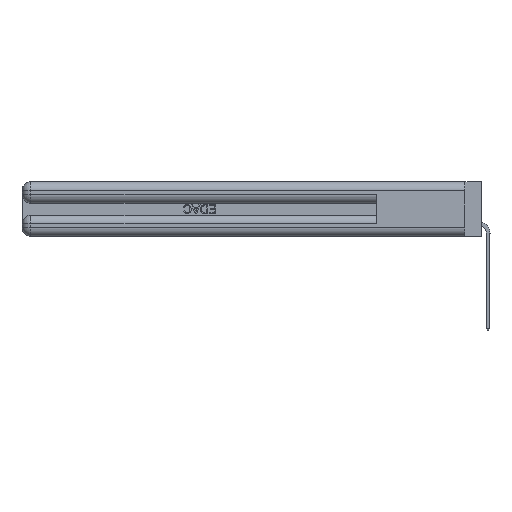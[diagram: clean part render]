
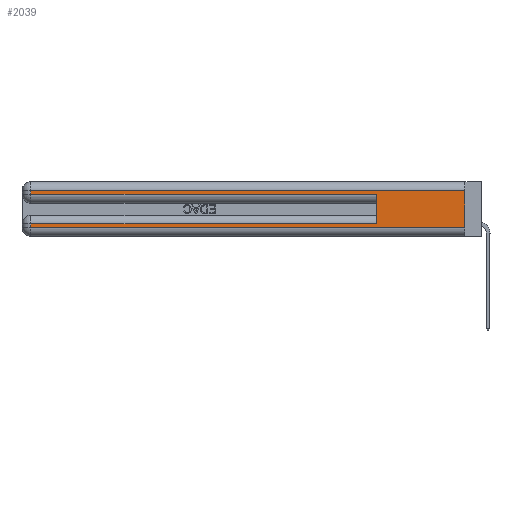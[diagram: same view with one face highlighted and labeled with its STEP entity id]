
A CAD part, left-side view. The second image highlights one B-rep face of the part: STEP entity #2039.
In plain terms, the highlighted planar face has unit normal (-1, 0, 0).
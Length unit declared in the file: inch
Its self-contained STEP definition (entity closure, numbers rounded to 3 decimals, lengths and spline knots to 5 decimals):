
#1283 = LINE ( 'NONE', #32755, #19797 ) ;
#1844 = EDGE_CURVE ( 'NONE', #20080, #29678, #5288, .T. ) ;
#2012 = DIRECTION ( 'NONE',  ( 0., 0., -1. ) ) ;
#2039 = ADVANCED_FACE ( 'NONE', ( #39711 ), #11212, .F. ) ;
#4358 = DIRECTION ( 'NONE',  ( 0., 1., 0. ) ) ;
#4381 = CARTESIAN_POINT ( 'NONE',  ( 0., 0., 0.285 ) ) ;
#4842 = LINE ( 'NONE', #4381, #40306 ) ;
#5288 = LINE ( 'NONE', #8274, #23747 ) ;
#5434 = EDGE_LOOP ( 'NONE', ( #35543, #8262, #37528, #19134, #39429, #38840, #17366, #28335 ) ) ;
#5841 = EDGE_CURVE ( 'NONE', #9917, #28536, #8396, .T. ) ;
#5960 = EDGE_CURVE ( 'NONE', #37163, #29678, #21373, .T. ) ;
#6861 = DIRECTION ( 'NONE',  ( 0., 0., -1. ) ) ;
#7276 = CARTESIAN_POINT ( 'NONE',  ( 0., 2.94, 0.37 ) ) ;
#8252 = CARTESIAN_POINT ( 'NONE',  ( 0., 2.94, 0.37 ) ) ;
#8262 = ORIENTED_EDGE ( 'NONE', *, *, #12371, .T. ) ;
#8274 = CARTESIAN_POINT ( 'NONE',  ( 0., 0., 0.37 ) ) ;
#8396 = LINE ( 'NONE', #16220, #25393 ) ;
#8474 = CARTESIAN_POINT ( 'NONE',  ( 0., 2.94, 0.06 ) ) ;
#9917 = VERTEX_POINT ( 'NONE', #32937 ) ;
#10785 = CARTESIAN_POINT ( 'NONE',  ( 0., 0., 0.31 ) ) ;
#11212 = PLANE ( 'NONE',  #32061 ) ;
#11316 = EDGE_CURVE ( 'NONE', #12801, #26693, #35589, .T. ) ;
#12371 = EDGE_CURVE ( 'NONE', #20080, #12801, #40641, .T. ) ;
#12664 = DIRECTION ( 'NONE',  ( 0., 0., -1. ) ) ;
#12801 = VERTEX_POINT ( 'NONE', #35189 ) ;
#15765 = CARTESIAN_POINT ( 'NONE',  ( 0., 0., 0.31 ) ) ;
#15889 = EDGE_CURVE ( 'NONE', #26693, #28536, #4842, .T. ) ;
#16038 = EDGE_CURVE ( 'NONE', #9917, #33114, #1283, .T. ) ;
#16220 = CARTESIAN_POINT ( 'NONE',  ( 0., 0.6, 0.145 ) ) ;
#17366 = ORIENTED_EDGE ( 'NONE', *, *, #32618, .T. ) ;
#18752 = VECTOR ( 'NONE', #6861, 39.37008 ) ;
#19134 = ORIENTED_EDGE ( 'NONE', *, *, #15889, .T. ) ;
#19797 = VECTOR ( 'NONE', #39759, 39.37008 ) ;
#20080 = VERTEX_POINT ( 'NONE', #15765 ) ;
#21373 = LINE ( 'NONE', #23965, #34326 ) ;
#22439 = CARTESIAN_POINT ( 'NONE',  ( 0., 0., 0.37 ) ) ;
#23747 = VECTOR ( 'NONE', #2012, 39.37008 ) ;
#23965 = CARTESIAN_POINT ( 'NONE',  ( 0., 0., 0.06 ) ) ;
#24268 = LINE ( 'NONE', #8252, #25289 ) ;
#24908 = DIRECTION ( 'NONE',  ( 1., 0., 0. ) ) ;
#25289 = VECTOR ( 'NONE', #36691, 39.37008 ) ;
#25393 = VECTOR ( 'NONE', #31012, 39.37008 ) ;
#26093 = CARTESIAN_POINT ( 'NONE',  ( 0., 0., 0.06 ) ) ;
#26693 = VERTEX_POINT ( 'NONE', #39604 ) ;
#28335 = ORIENTED_EDGE ( 'NONE', *, *, #5960, .T. ) ;
#28536 = VERTEX_POINT ( 'NONE', #28780 ) ;
#28780 = CARTESIAN_POINT ( 'NONE',  ( 0., 0.6, 0.285 ) ) ;
#29539 = CARTESIAN_POINT ( 'NONE',  ( 0., 2.94, 0.085 ) ) ;
#29678 = VERTEX_POINT ( 'NONE', #26093 ) ;
#30105 = DIRECTION ( 'NONE',  ( 0., -1., 0. ) ) ;
#30904 = DIRECTION ( 'NONE',  ( 0., -1., 0. ) ) ;
#31012 = DIRECTION ( 'NONE',  ( 0., 0., 1. ) ) ;
#32061 = AXIS2_PLACEMENT_3D ( 'NONE', #22439, #24908, #12664 ) ;
#32096 = VECTOR ( 'NONE', #4358, 39.37008 ) ;
#32618 = EDGE_CURVE ( 'NONE', #33114, #37163, #24268, .T. ) ;
#32755 = CARTESIAN_POINT ( 'NONE',  ( 0., 0., 0.085 ) ) ;
#32937 = CARTESIAN_POINT ( 'NONE',  ( 0., 0.6, 0.085 ) ) ;
#33114 = VERTEX_POINT ( 'NONE', #29539 ) ;
#34326 = VECTOR ( 'NONE', #30105, 39.37008 ) ;
#35189 = CARTESIAN_POINT ( 'NONE',  ( 0., 2.94, 0.31 ) ) ;
#35543 = ORIENTED_EDGE ( 'NONE', *, *, #1844, .F. ) ;
#35589 = LINE ( 'NONE', #7276, #18752 ) ;
#36691 = DIRECTION ( 'NONE',  ( 0., 0., -1. ) ) ;
#37163 = VERTEX_POINT ( 'NONE', #8474 ) ;
#37528 = ORIENTED_EDGE ( 'NONE', *, *, #11316, .T. ) ;
#38840 = ORIENTED_EDGE ( 'NONE', *, *, #16038, .T. ) ;
#39429 = ORIENTED_EDGE ( 'NONE', *, *, #5841, .F. ) ;
#39604 = CARTESIAN_POINT ( 'NONE',  ( 0., 2.94, 0.285 ) ) ;
#39711 = FACE_OUTER_BOUND ( 'NONE', #5434, .T. ) ;
#39759 = DIRECTION ( 'NONE',  ( 0., 1., 0. ) ) ;
#40306 = VECTOR ( 'NONE', #30904, 39.37008 ) ;
#40641 = LINE ( 'NONE', #10785, #32096 ) ;
